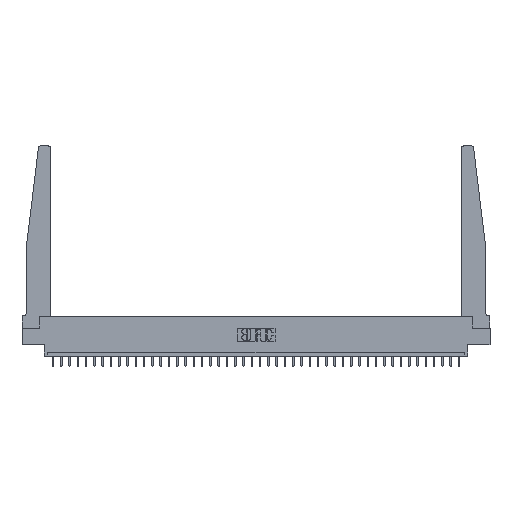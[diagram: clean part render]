
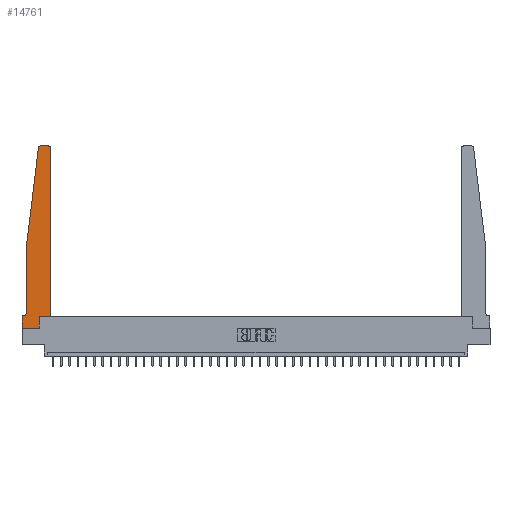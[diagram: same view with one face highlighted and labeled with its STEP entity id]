
A CAD part, top view. The second image highlights one B-rep face of the part: STEP entity #14761.
In plain terms, the highlighted planar face has unit normal (0, 0, 1).
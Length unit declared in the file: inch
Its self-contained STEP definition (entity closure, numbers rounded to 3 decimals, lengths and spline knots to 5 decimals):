
#137 = ORIENTED_EDGE ( 'NONE', *, *, #32367, .T. ) ;
#706 = VECTOR ( 'NONE', #1258, 39.37008 ) ;
#1106 = DIRECTION ( 'NONE',  ( 1., 0., 0. ) ) ;
#1258 = DIRECTION ( 'NONE',  ( -1., 0., 0. ) ) ;
#1270 = CIRCLE ( 'NONE', #15823, 0.03 ) ;
#1286 = CARTESIAN_POINT ( 'NONE',  ( 0., 0., 0.37 ) ) ;
#1692 = DIRECTION ( 'NONE',  ( 0., 0., 1. ) ) ;
#2201 = ORIENTED_EDGE ( 'NONE', *, *, #30153, .T. ) ;
#2638 = LINE ( 'NONE', #22614, #9796 ) ;
#2692 = ORIENTED_EDGE ( 'NONE', *, *, #6539, .T. ) ;
#3805 = VECTOR ( 'NONE', #17804, 39.37008 ) ;
#3809 = EDGE_LOOP ( 'NONE', ( #15939, #19715, #9387, #18036, #10293, #137, #9774, #2692, #13404, #28034, #25267, #2201 ) ) ;
#5230 = DIRECTION ( 'NONE',  ( 1., 0., 0. ) ) ;
#5360 = VERTEX_POINT ( 'NONE', #31985 ) ;
#5514 = CARTESIAN_POINT ( 'NONE',  ( 0.24675, 2.72367, 0.37 ) ) ;
#6539 = EDGE_CURVE ( 'NONE', #25908, #13490, #11003, .T. ) ;
#6841 = LINE ( 'NONE', #29182, #18281 ) ;
#7520 = EDGE_CURVE ( 'NONE', #27463, #25908, #12162, .T. ) ;
#7797 = LINE ( 'NONE', #33877, #28475 ) ;
#7919 = VECTOR ( 'NONE', #1106, 39.37008 ) ;
#9387 = ORIENTED_EDGE ( 'NONE', *, *, #33464, .T. ) ;
#9390 = CARTESIAN_POINT ( 'NONE',  ( 0.425, 0.18, 0.37 ) ) ;
#9407 = CARTESIAN_POINT ( 'NONE',  ( 0., 0.1875, 0.37 ) ) ;
#9476 = VECTOR ( 'NONE', #16080, 39.37008 ) ;
#9774 = ORIENTED_EDGE ( 'NONE', *, *, #7520, .T. ) ;
#9796 = VECTOR ( 'NONE', #20033, 39.37008 ) ;
#9802 = DIRECTION ( 'NONE',  ( 0., -1., 0. ) ) ;
#9850 = CARTESIAN_POINT ( 'NONE',  ( 0.2605, 0., 0.37 ) ) ;
#10039 = VERTEX_POINT ( 'NONE', #32926 ) ;
#10293 = ORIENTED_EDGE ( 'NONE', *, *, #29538, .T. ) ;
#10552 = VERTEX_POINT ( 'NONE', #30275 ) ;
#10882 = LINE ( 'NONE', #27053, #706 ) ;
#11003 = LINE ( 'NONE', #1286, #3805 ) ;
#11773 = CARTESIAN_POINT ( 'NONE',  ( 0.395, 2.75, 0.37 ) ) ;
#12116 = EDGE_CURVE ( 'NONE', #18244, #10552, #16641, .T. ) ;
#12162 = LINE ( 'NONE', #17691, #15526 ) ;
#12472 = CARTESIAN_POINT ( 'NONE',  ( 0.015, 0.1875, 0.37 ) ) ;
#12593 = CIRCLE ( 'NONE', #26262, 0.03 ) ;
#12681 = CARTESIAN_POINT ( 'NONE',  ( 0.395, 2.72, 0.37 ) ) ;
#13063 = EDGE_CURVE ( 'NONE', #10039, #5360, #6841, .T. ) ;
#13404 = ORIENTED_EDGE ( 'NONE', *, *, #33706, .T. ) ;
#13490 = VERTEX_POINT ( 'NONE', #9850 ) ;
#13719 = VECTOR ( 'NONE', #14048, 39.37008 ) ;
#14048 = DIRECTION ( 'NONE',  ( -0.122, -0.992, 0. ) ) ;
#14761 = ADVANCED_FACE ( 'NONE', ( #23201 ), #18496, .T. ) ;
#14909 = DIRECTION ( 'NONE',  ( 1., 0., 0. ) ) ;
#15526 = VECTOR ( 'NONE', #9802, 39.37008 ) ;
#15823 = AXIS2_PLACEMENT_3D ( 'NONE', #12681, #1692, #14909 ) ;
#15939 = ORIENTED_EDGE ( 'NONE', *, *, #12116, .T. ) ;
#16080 = DIRECTION ( 'NONE',  ( -1., 0., 0. ) ) ;
#16641 = LINE ( 'NONE', #31527, #9476 ) ;
#17248 = DIRECTION ( 'NONE',  ( -1., 0., 0. ) ) ;
#17691 = CARTESIAN_POINT ( 'NONE',  ( 0., 0., 0.37 ) ) ;
#17804 = DIRECTION ( 'NONE',  ( 1., 0., 0. ) ) ;
#18036 = ORIENTED_EDGE ( 'NONE', *, *, #24629, .T. ) ;
#18244 = VERTEX_POINT ( 'NONE', #11773 ) ;
#18281 = VECTOR ( 'NONE', #31889, 39.37008 ) ;
#18331 = VERTEX_POINT ( 'NONE', #27800 ) ;
#18496 = PLANE ( 'NONE',  #22339 ) ;
#18691 = CARTESIAN_POINT ( 'NONE',  ( 0.065, 1.25, 0.37 ) ) ;
#19172 = EDGE_CURVE ( 'NONE', #10552, #31652, #12593, .T. ) ;
#19614 = CARTESIAN_POINT ( 'NONE',  ( 0.015, 0.2375, 0.37 ) ) ;
#19715 = ORIENTED_EDGE ( 'NONE', *, *, #19172, .T. ) ;
#20033 = DIRECTION ( 'NONE',  ( 0., -1., 0. ) ) ;
#21161 = CARTESIAN_POINT ( 'NONE',  ( 0., 0.1875, 0.37 ) ) ;
#21628 = DIRECTION ( 'NONE',  ( 0., 0., 1. ) ) ;
#22339 = AXIS2_PLACEMENT_3D ( 'NONE', #21161, #29996, #28546 ) ;
#22507 = VERTEX_POINT ( 'NONE', #12472 ) ;
#22614 = CARTESIAN_POINT ( 'NONE',  ( 0.065, 1.25, 0.37 ) ) ;
#23001 = VERTEX_POINT ( 'NONE', #31165 ) ;
#23201 = FACE_OUTER_BOUND ( 'NONE', #3809, .T. ) ;
#23560 = DIRECTION ( 'NONE',  ( 0., 1., 0. ) ) ;
#24116 = CIRCLE ( 'NONE', #28212, 0.05 ) ;
#24629 = EDGE_CURVE ( 'NONE', #33219, #23001, #2638, .T. ) ;
#25267 = ORIENTED_EDGE ( 'NONE', *, *, #13063, .T. ) ;
#25557 = LINE ( 'NONE', #30178, #13719 ) ;
#25908 = VERTEX_POINT ( 'NONE', #27483 ) ;
#26262 = AXIS2_PLACEMENT_3D ( 'NONE', #29491, #21628, #5230 ) ;
#27053 = CARTESIAN_POINT ( 'NONE',  ( 0.065, 0.1875, 0.37 ) ) ;
#27463 = VERTEX_POINT ( 'NONE', #9407 ) ;
#27483 = CARTESIAN_POINT ( 'NONE',  ( 0., 0., 0.37 ) ) ;
#27800 = CARTESIAN_POINT ( 'NONE',  ( 0.2605, 0.18, 0.37 ) ) ;
#28034 = ORIENTED_EDGE ( 'NONE', *, *, #31874, .T. ) ;
#28212 = AXIS2_PLACEMENT_3D ( 'NONE', #19614, #33317, #17248 ) ;
#28475 = VECTOR ( 'NONE', #23560, 39.37008 ) ;
#28546 = DIRECTION ( 'NONE',  ( 1., 0., 0. ) ) ;
#29036 = LINE ( 'NONE', #9390, #7919 ) ;
#29182 = CARTESIAN_POINT ( 'NONE',  ( 0.425, 0.18, 0.37 ) ) ;
#29491 = CARTESIAN_POINT ( 'NONE',  ( 0.27653, 2.72, 0.37 ) ) ;
#29538 = EDGE_CURVE ( 'NONE', #23001, #22507, #24116, .T. ) ;
#29996 = DIRECTION ( 'NONE',  ( 0., 0., 1. ) ) ;
#30153 = EDGE_CURVE ( 'NONE', #5360, #18244, #1270, .T. ) ;
#30178 = CARTESIAN_POINT ( 'NONE',  ( 0.065, 1.25, 0.37 ) ) ;
#30275 = CARTESIAN_POINT ( 'NONE',  ( 0.27653, 2.75, 0.37 ) ) ;
#31165 = CARTESIAN_POINT ( 'NONE',  ( 0.065, 0.2375, 0.37 ) ) ;
#31527 = CARTESIAN_POINT ( 'NONE',  ( 0.25, 2.75, 0.37 ) ) ;
#31652 = VERTEX_POINT ( 'NONE', #5514 ) ;
#31874 = EDGE_CURVE ( 'NONE', #18331, #10039, #29036, .T. ) ;
#31889 = DIRECTION ( 'NONE',  ( 0., 1., 0. ) ) ;
#31985 = CARTESIAN_POINT ( 'NONE',  ( 0.425, 2.72, 0.37 ) ) ;
#32367 = EDGE_CURVE ( 'NONE', #22507, #27463, #10882, .T. ) ;
#32926 = CARTESIAN_POINT ( 'NONE',  ( 0.425, 0.18, 0.37 ) ) ;
#33219 = VERTEX_POINT ( 'NONE', #18691 ) ;
#33317 = DIRECTION ( 'NONE',  ( 0., 0., -1. ) ) ;
#33464 = EDGE_CURVE ( 'NONE', #31652, #33219, #25557, .T. ) ;
#33706 = EDGE_CURVE ( 'NONE', #13490, #18331, #7797, .T. ) ;
#33877 = CARTESIAN_POINT ( 'NONE',  ( 0.2605, 0.18, 0.37 ) ) ;
